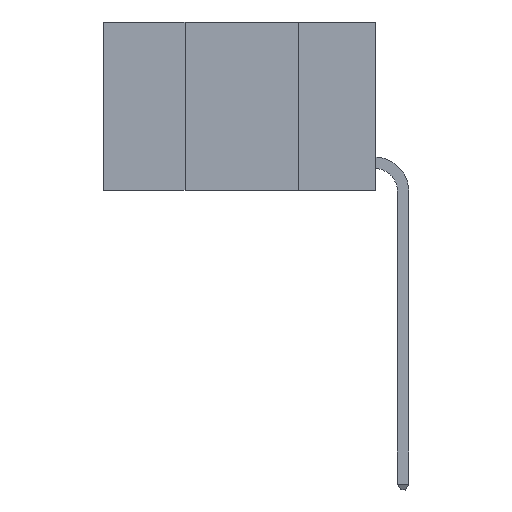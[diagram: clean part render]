
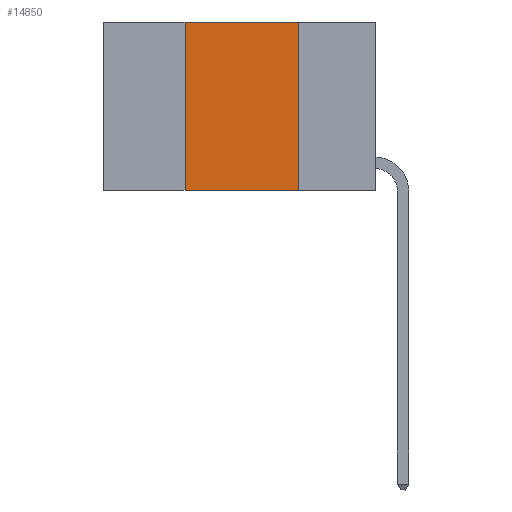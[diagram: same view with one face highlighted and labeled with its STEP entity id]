
A CAD part, left-side view. The second image highlights one B-rep face of the part: STEP entity #14850.
In plain terms, the highlighted planar face has unit normal (-1, 0, 0).
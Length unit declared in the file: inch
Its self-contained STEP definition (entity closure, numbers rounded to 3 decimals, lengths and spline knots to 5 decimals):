
#102 = CARTESIAN_POINT ( 'NONE',  ( 0., 0.6, 0. ) ) ;
#781 = EDGE_LOOP ( 'NONE', ( #5220, #20581, #8933, #9355 ) ) ;
#851 = CARTESIAN_POINT ( 'NONE',  ( 0., 0.17, -0.37 ) ) ;
#1585 = DIRECTION ( 'NONE',  ( 0., -1., 0. ) ) ;
#1776 = VERTEX_POINT ( 'NONE', #6121 ) ;
#1874 = DIRECTION ( 'NONE',  ( 1., 0., 0. ) ) ;
#2192 = DIRECTION ( 'NONE',  ( 0., 0., -1. ) ) ;
#3296 = LINE ( 'NONE', #102, #5155 ) ;
#3799 = PLANE ( 'NONE',  #12966 ) ;
#3800 = EDGE_CURVE ( 'NONE', #5069, #1776, #3296, .T. ) ;
#4964 = FACE_OUTER_BOUND ( 'NONE', #781, .T. ) ;
#5069 = VERTEX_POINT ( 'NONE', #8822 ) ;
#5155 = VECTOR ( 'NONE', #1585, 39.37008 ) ;
#5220 = ORIENTED_EDGE ( 'NONE', *, *, #9506, .F. ) ;
#5272 = DIRECTION ( 'NONE',  ( 0., 0., 1. ) ) ;
#5863 = VERTEX_POINT ( 'NONE', #8130 ) ;
#6093 = CARTESIAN_POINT ( 'NONE',  ( 0., 0.17, 0. ) ) ;
#6121 = CARTESIAN_POINT ( 'NONE',  ( 0., 0.17, 0. ) ) ;
#6731 = VECTOR ( 'NONE', #12634, 39.37008 ) ;
#7081 = LINE ( 'NONE', #13415, #9749 ) ;
#8130 = CARTESIAN_POINT ( 'NONE',  ( 0., 0.42, -0.37 ) ) ;
#8706 = EDGE_CURVE ( 'NONE', #5863, #5069, #7081, .T. ) ;
#8822 = CARTESIAN_POINT ( 'NONE',  ( 0., 0.42, 0. ) ) ;
#8933 = ORIENTED_EDGE ( 'NONE', *, *, #8706, .F. ) ;
#9355 = ORIENTED_EDGE ( 'NONE', *, *, #15948, .T. ) ;
#9506 = EDGE_CURVE ( 'NONE', #1776, #17182, #20782, .T. ) ;
#9749 = VECTOR ( 'NONE', #5272, 39.37008 ) ;
#12634 = DIRECTION ( 'NONE',  ( 0., 0., -1. ) ) ;
#12966 = AXIS2_PLACEMENT_3D ( 'NONE', #18346, #1874, #2192 ) ;
#13415 = CARTESIAN_POINT ( 'NONE',  ( 0., 0.42, 0. ) ) ;
#14850 = ADVANCED_FACE ( 'NONE', ( #4964 ), #3799, .F. ) ;
#15124 = VECTOR ( 'NONE', #17406, 39.37008 ) ;
#15677 = CARTESIAN_POINT ( 'NONE',  ( 0., 0.6, -0.37 ) ) ;
#15948 = EDGE_CURVE ( 'NONE', #5863, #17182, #19120, .T. ) ;
#17182 = VERTEX_POINT ( 'NONE', #851 ) ;
#17406 = DIRECTION ( 'NONE',  ( 0., -1., 0. ) ) ;
#18346 = CARTESIAN_POINT ( 'NONE',  ( 0., 0.6, 0. ) ) ;
#19120 = LINE ( 'NONE', #15677, #15124 ) ;
#20581 = ORIENTED_EDGE ( 'NONE', *, *, #3800, .F. ) ;
#20782 = LINE ( 'NONE', #6093, #6731 ) ;
